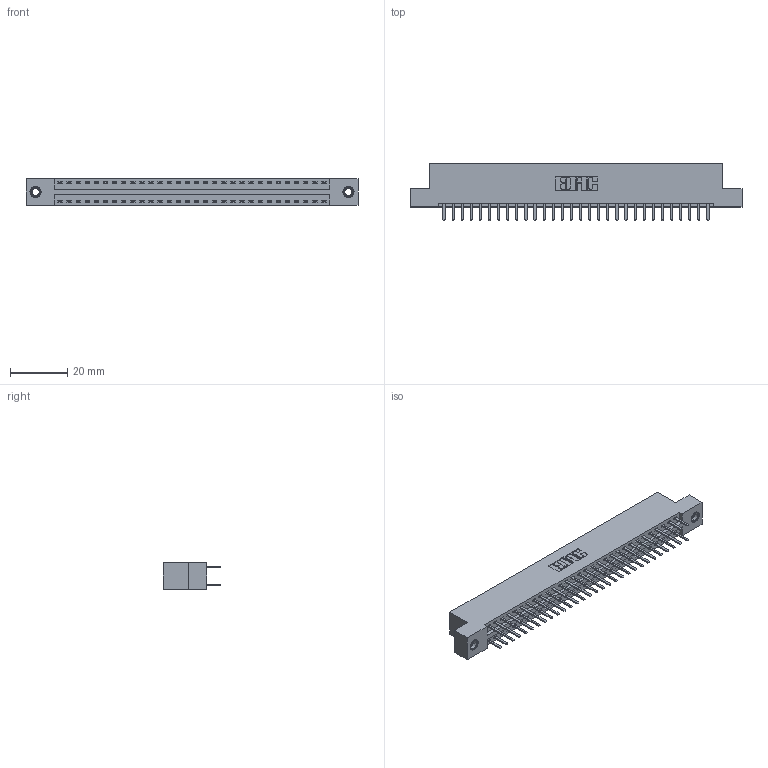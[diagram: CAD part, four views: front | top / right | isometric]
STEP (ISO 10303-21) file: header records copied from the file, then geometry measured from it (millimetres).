
FILE_DESCRIPTION (( 'STEP AP203' ), '1' );
FILE_NAME ('346-060-520-207.STEP', '2022-05-21T10:19:45', ( '' ), ( '' ), 'SwSTEP 2.0', 'SolidWorks 2020', '' );
FILE_SCHEMA (( 'CONFIG_CONTROL_DESIGN' ));
Length unit declared in the file: inch
Products named in the file (4): 346 Part_Flush Mounting Lugs - 0.156 Dia-TI; 345-250-001_345-250-005-103; 345-292-001_345-293-120; 346-060-520-207
Assembly tree (63 placements, depth 2):
  346-060-520-207
    346 Part_Flush Mounting Lugs - 0.156 Dia-TI
    345-292-001_345-293-120  x60
    345-250-001_345-250-005-103  x2
Bounding box: 115.82 x 20.02 x 9.4 mm (x, y, z)
Volume: 11161.2 mm3; surface area: 15125.1 mm2
Topology: 63 solids, 63 shells, 3542 faces, 10245 edges, 6662 vertices
Faces by surface type: plane 2328, cylinder 1198, cone 12, torus 4
Entity records: 22494 total; most frequent: CARTESIAN_POINT 3719, ORIENTED_EDGE 3634, DIRECTION 3343, EDGE_CURVE 1817, VECTOR 1541, LINE 1541, VERTEX_POINT 1204, AXIS2_PLACEMENT_3D 901
